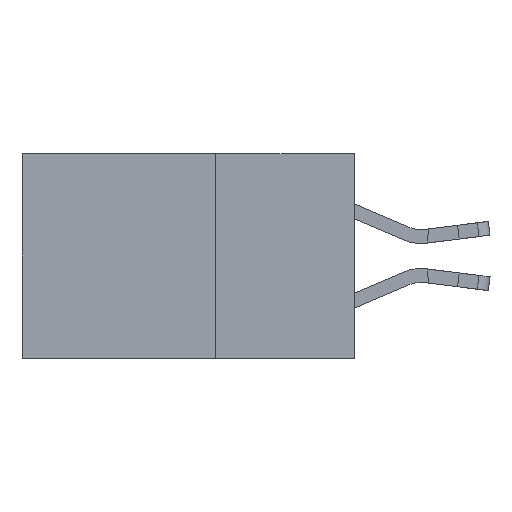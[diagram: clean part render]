
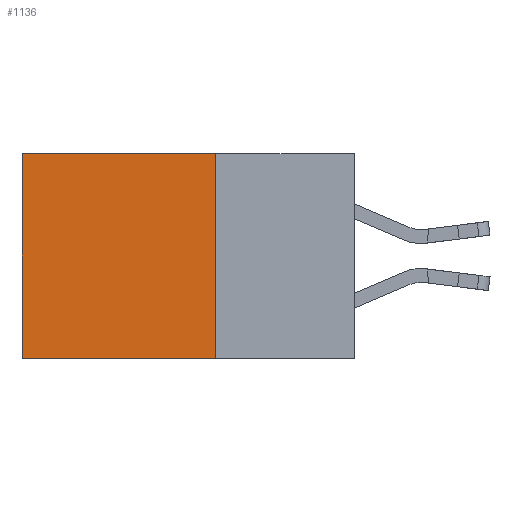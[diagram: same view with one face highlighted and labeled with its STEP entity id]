
A CAD part, left-side view. The second image highlights one B-rep face of the part: STEP entity #1136.
In plain terms, the highlighted planar face has unit normal (-1, 0, 0).
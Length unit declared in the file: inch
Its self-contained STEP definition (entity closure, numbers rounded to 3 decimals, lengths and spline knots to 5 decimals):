
#443 = VERTEX_POINT ( 'NONE', #10672 ) ;
#1136 = ADVANCED_FACE ( 'NONE', ( #14098 ), #10570, .F. ) ;
#1885 = VECTOR ( 'NONE', #6803, 39.37008 ) ;
#2345 = EDGE_CURVE ( 'NONE', #24663, #11582, #23818, .T. ) ;
#2383 = EDGE_CURVE ( 'NONE', #443, #14583, #27297, .T. ) ;
#3747 = DIRECTION ( 'NONE',  ( 0., 0., -1. ) ) ;
#3911 = CARTESIAN_POINT ( 'NONE',  ( 0.298, 0.25, 0. ) ) ;
#4059 = AXIS2_PLACEMENT_3D ( 'NONE', #12630, #17130, #3747 ) ;
#4292 = ORIENTED_EDGE ( 'NONE', *, *, #2383, .T. ) ;
#5661 = VECTOR ( 'NONE', #12070, 39.37008 ) ;
#6697 = EDGE_CURVE ( 'NONE', #11582, #14583, #17616, .T. ) ;
#6803 = DIRECTION ( 'NONE',  ( 0., 1., 0. ) ) ;
#6836 = LINE ( 'NONE', #3911, #25350 ) ;
#6896 = ORIENTED_EDGE ( 'NONE', *, *, #17280, .T. ) ;
#7224 = EDGE_LOOP ( 'NONE', ( #4292, #25456, #9443, #6896 ) ) ;
#9042 = CARTESIAN_POINT ( 'NONE',  ( 0.298, 0.25, -0.37 ) ) ;
#9443 = ORIENTED_EDGE ( 'NONE', *, *, #2345, .F. ) ;
#9802 = CARTESIAN_POINT ( 'NONE',  ( 0.298, 0.25, 0. ) ) ;
#10545 = DIRECTION ( 'NONE',  ( 0., 1., 0. ) ) ;
#10570 = PLANE ( 'NONE',  #4059 ) ;
#10672 = CARTESIAN_POINT ( 'NONE',  ( 0.298, 0.6, 0. ) ) ;
#11582 = VERTEX_POINT ( 'NONE', #23382 ) ;
#12070 = DIRECTION ( 'NONE',  ( 0., 0., -1. ) ) ;
#12630 = CARTESIAN_POINT ( 'NONE',  ( 0.298, 0.25, 0. ) ) ;
#13710 = VECTOR ( 'NONE', #25746, 39.37008 ) ;
#14098 = FACE_OUTER_BOUND ( 'NONE', #7224, .T. ) ;
#14228 = CARTESIAN_POINT ( 'NONE',  ( 0.298, 0.6, 0. ) ) ;
#14583 = VERTEX_POINT ( 'NONE', #16445 ) ;
#16445 = CARTESIAN_POINT ( 'NONE',  ( 0.298, 0.6, -0.37 ) ) ;
#17130 = DIRECTION ( 'NONE',  ( 1., 0., 0. ) ) ;
#17280 = EDGE_CURVE ( 'NONE', #24663, #443, #6836, .T. ) ;
#17616 = LINE ( 'NONE', #9042, #1885 ) ;
#23360 = CARTESIAN_POINT ( 'NONE',  ( 0.298, 0.25, 0. ) ) ;
#23382 = CARTESIAN_POINT ( 'NONE',  ( 0.298, 0.25, -0.37 ) ) ;
#23818 = LINE ( 'NONE', #9802, #5661 ) ;
#24663 = VERTEX_POINT ( 'NONE', #23360 ) ;
#25350 = VECTOR ( 'NONE', #10545, 39.37008 ) ;
#25456 = ORIENTED_EDGE ( 'NONE', *, *, #6697, .F. ) ;
#25746 = DIRECTION ( 'NONE',  ( 0., 0., -1. ) ) ;
#27297 = LINE ( 'NONE', #14228, #13710 ) ;
